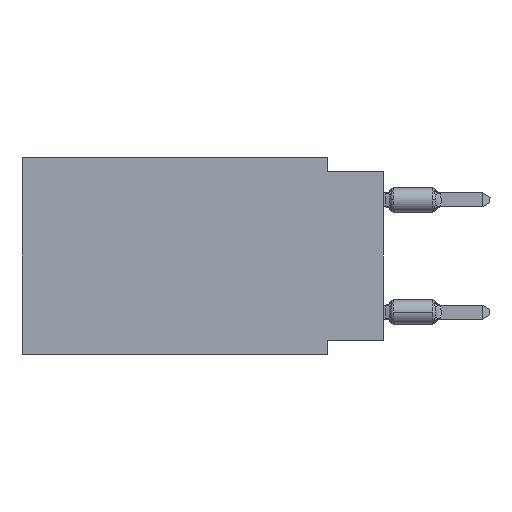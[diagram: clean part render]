
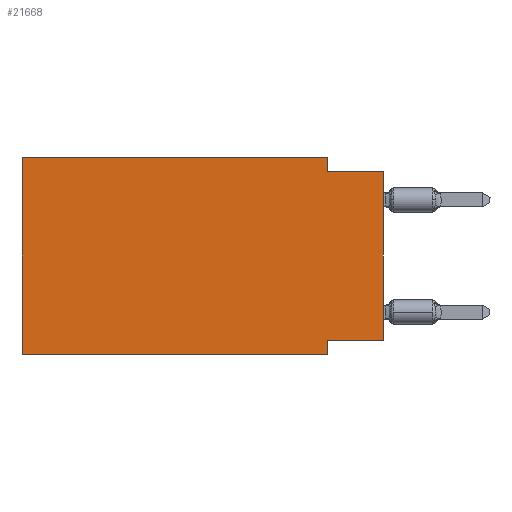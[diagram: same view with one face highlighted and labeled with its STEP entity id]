
A CAD part, left-side view. The second image highlights one B-rep face of the part: STEP entity #21668.
In plain terms, the highlighted planar face has unit normal (-1, 0, 0).
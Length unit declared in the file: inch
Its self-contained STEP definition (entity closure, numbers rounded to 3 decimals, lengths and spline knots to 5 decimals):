
#952 = VECTOR ( 'NONE', #28894, 39.37008 ) ;
#2664 = DIRECTION ( 'NONE',  ( 0., -1., 0. ) ) ;
#2666 = VECTOR ( 'NONE', #9083, 39.37008 ) ;
#2830 = CARTESIAN_POINT ( 'NONE',  ( 0., 0.1, -0.325 ) ) ;
#2849 = VECTOR ( 'NONE', #4465, 39.37008 ) ;
#3341 = CARTESIAN_POINT ( 'NONE',  ( 0., 0., 0. ) ) ;
#3838 = EDGE_CURVE ( 'NONE', #16767, #23544, #32130, .T. ) ;
#4071 = EDGE_CURVE ( 'NONE', #14200, #5165, #7496, .T. ) ;
#4080 = CARTESIAN_POINT ( 'NONE',  ( 0., 0., -0.325 ) ) ;
#4450 = CARTESIAN_POINT ( 'NONE',  ( 0., 0.1, -0.025 ) ) ;
#4465 = DIRECTION ( 'NONE',  ( 0., -1., 0. ) ) ;
#4652 = DIRECTION ( 'NONE',  ( 0., 1., 0. ) ) ;
#4716 = ORIENTED_EDGE ( 'NONE', *, *, #36944, .T. ) ;
#5165 = VERTEX_POINT ( 'NONE', #38849 ) ;
#5707 = ORIENTED_EDGE ( 'NONE', *, *, #31277, .T. ) ;
#6258 = EDGE_CURVE ( 'NONE', #23544, #23011, #8965, .T. ) ;
#7496 = LINE ( 'NONE', #31460, #22203 ) ;
#7849 = LINE ( 'NONE', #8237, #2849 ) ;
#8110 = EDGE_CURVE ( 'NONE', #5165, #16767, #23010, .T. ) ;
#8237 = CARTESIAN_POINT ( 'NONE',  ( 0., 0.645, -0.35 ) ) ;
#8965 = LINE ( 'NONE', #12094, #30461 ) ;
#9083 = DIRECTION ( 'NONE',  ( 0., 0., 1. ) ) ;
#9341 = ORIENTED_EDGE ( 'NONE', *, *, #18215, .F. ) ;
#9573 = ORIENTED_EDGE ( 'NONE', *, *, #8110, .F. ) ;
#9739 = LINE ( 'NONE', #15426, #15620 ) ;
#11463 = ORIENTED_EDGE ( 'NONE', *, *, #4071, .F. ) ;
#11464 = AXIS2_PLACEMENT_3D ( 'NONE', #17660, #23222, #17487 ) ;
#12094 = CARTESIAN_POINT ( 'NONE',  ( 0., 0., -0.025 ) ) ;
#12257 = VERTEX_POINT ( 'NONE', #32442 ) ;
#13131 = CARTESIAN_POINT ( 'NONE',  ( 0., 0.1, 0. ) ) ;
#14025 = VERTEX_POINT ( 'NONE', #2830 ) ;
#14048 = VECTOR ( 'NONE', #26605, 39.37008 ) ;
#14171 = PLANE ( 'NONE',  #11464 ) ;
#14179 = ORIENTED_EDGE ( 'NONE', *, *, #6258, .F. ) ;
#14200 = VERTEX_POINT ( 'NONE', #17975 ) ;
#14353 = FACE_OUTER_BOUND ( 'NONE', #19368, .T. ) ;
#14913 = ORIENTED_EDGE ( 'NONE', *, *, #3838, .F. ) ;
#15426 = CARTESIAN_POINT ( 'NONE',  ( 0., 0.1, -0.35 ) ) ;
#15620 = VECTOR ( 'NONE', #27426, 39.37008 ) ;
#16767 = VERTEX_POINT ( 'NONE', #13131 ) ;
#17487 = DIRECTION ( 'NONE',  ( 0., 0., -1. ) ) ;
#17660 = CARTESIAN_POINT ( 'NONE',  ( 0., 0.645, 0. ) ) ;
#17975 = CARTESIAN_POINT ( 'NONE',  ( 0., 0.645, -0.35 ) ) ;
#18215 = EDGE_CURVE ( 'NONE', #34449, #14025, #26112, .T. ) ;
#19368 = EDGE_LOOP ( 'NONE', ( #5707, #14179, #14913, #9573, #11463, #4716, #24558, #9341 ) ) ;
#20900 = CARTESIAN_POINT ( 'NONE',  ( 0., 0.1, 0. ) ) ;
#21668 = ADVANCED_FACE ( 'NONE', ( #14353 ), #14171, .F. ) ;
#22203 = VECTOR ( 'NONE', #22230, 39.37008 ) ;
#22230 = DIRECTION ( 'NONE',  ( 0., 0., 1. ) ) ;
#23010 = LINE ( 'NONE', #25947, #952 ) ;
#23011 = VERTEX_POINT ( 'NONE', #33426 ) ;
#23222 = DIRECTION ( 'NONE',  ( 1., 0., 0. ) ) ;
#23544 = VERTEX_POINT ( 'NONE', #4450 ) ;
#24558 = ORIENTED_EDGE ( 'NONE', *, *, #26068, .F. ) ;
#25947 = CARTESIAN_POINT ( 'NONE',  ( 0., 0.645, 0. ) ) ;
#26068 = EDGE_CURVE ( 'NONE', #14025, #12257, #9739, .T. ) ;
#26112 = LINE ( 'NONE', #29242, #34011 ) ;
#26605 = DIRECTION ( 'NONE',  ( 0., 0., -1. ) ) ;
#27148 = LINE ( 'NONE', #3341, #2666 ) ;
#27426 = DIRECTION ( 'NONE',  ( 0., 0., -1. ) ) ;
#28894 = DIRECTION ( 'NONE',  ( 0., -1., 0. ) ) ;
#29242 = CARTESIAN_POINT ( 'NONE',  ( 0., 0., -0.325 ) ) ;
#30461 = VECTOR ( 'NONE', #2664, 39.37008 ) ;
#31277 = EDGE_CURVE ( 'NONE', #34449, #23011, #27148, .T. ) ;
#31460 = CARTESIAN_POINT ( 'NONE',  ( 0., 0.645, 0. ) ) ;
#32130 = LINE ( 'NONE', #20900, #14048 ) ;
#32442 = CARTESIAN_POINT ( 'NONE',  ( 0., 0.1, -0.35 ) ) ;
#33426 = CARTESIAN_POINT ( 'NONE',  ( 0., 0., -0.025 ) ) ;
#34011 = VECTOR ( 'NONE', #4652, 39.37008 ) ;
#34449 = VERTEX_POINT ( 'NONE', #4080 ) ;
#36944 = EDGE_CURVE ( 'NONE', #14200, #12257, #7849, .T. ) ;
#38849 = CARTESIAN_POINT ( 'NONE',  ( 0., 0.645, 0. ) ) ;
